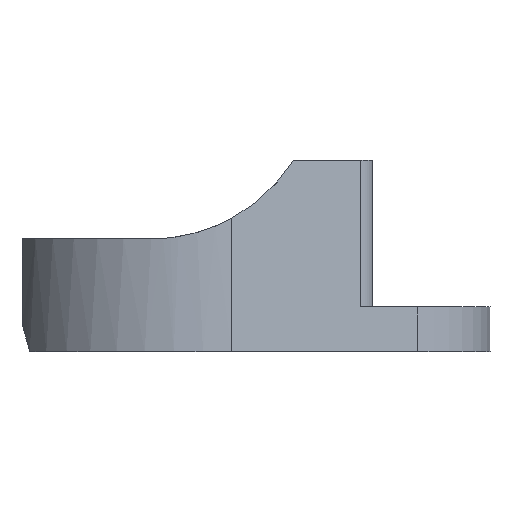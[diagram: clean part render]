
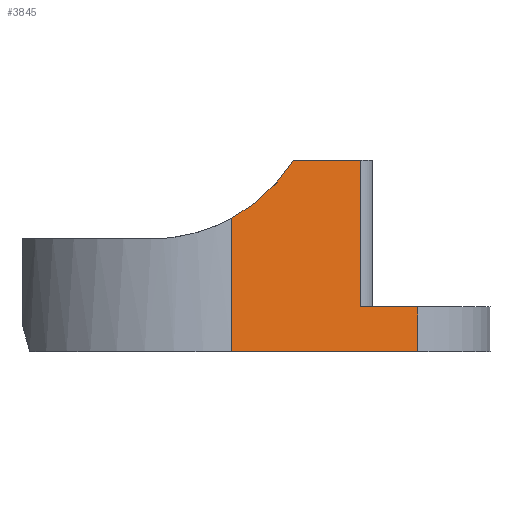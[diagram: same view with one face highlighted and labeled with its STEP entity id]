
A CAD part, left-side view. The second image highlights one B-rep face of the part: STEP entity #3845.
In plain terms, the highlighted planar face has unit normal (-0.95, -0.313, 0).
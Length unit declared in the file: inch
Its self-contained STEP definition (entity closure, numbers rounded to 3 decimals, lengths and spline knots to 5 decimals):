
#23=ELLIPSE('',#4035,0.78969,0.75);
#34=PLANE('',#4072);
#264=FACE_OUTER_BOUND('',#473,.T.);
#473=EDGE_LOOP('',(#3395,#3396,#3397,#3398,#3399,#3400,#3401));
#1074=LINE('',#12068,#1229);
#1077=LINE('',#16087,#1232);
#1079=LINE('',#16093,#1234);
#1080=LINE('',#16094,#1235);
#1081=LINE('',#16095,#1236);
#1082=LINE('',#16096,#1237);
#1229=VECTOR('',#4589,0.3937);
#1232=VECTOR('',#4628,0.3937);
#1234=VECTOR('',#4634,0.3937);
#1235=VECTOR('',#4635,0.3937);
#1236=VECTOR('',#4636,0.3937);
#1237=VECTOR('',#4637,0.3937);
#1628=VERTEX_POINT('',#11942);
#1629=VERTEX_POINT('',#11951);
#1638=VERTEX_POINT('',#12065);
#1639=VERTEX_POINT('',#12067);
#1644=VERTEX_POINT('',#16084);
#1645=VERTEX_POINT('',#16086);
#1647=VERTEX_POINT('',#16092);
#2174=EDGE_CURVE('',#1628,#1629,#23,.T.);
#2200=EDGE_CURVE('',#1638,#1639,#1074,.T.);
#2239=EDGE_CURVE('',#1644,#1645,#1077,.T.);
#2242=EDGE_CURVE('',#1645,#1647,#1079,.T.);
#2243=EDGE_CURVE('',#1629,#1644,#1080,.T.);
#2244=EDGE_CURVE('',#1639,#1628,#1081,.T.);
#2245=EDGE_CURVE('',#1638,#1647,#1082,.T.);
#3395=ORIENTED_EDGE('',*,*,#2242,.F.);
#3396=ORIENTED_EDGE('',*,*,#2239,.F.);
#3397=ORIENTED_EDGE('',*,*,#2243,.F.);
#3398=ORIENTED_EDGE('',*,*,#2174,.F.);
#3399=ORIENTED_EDGE('',*,*,#2244,.F.);
#3400=ORIENTED_EDGE('',*,*,#2200,.F.);
#3401=ORIENTED_EDGE('',*,*,#2245,.T.);
#3845=ADVANCED_FACE('',(#264),#34,.F.);
#4035=AXIS2_PLACEMENT_3D('',#11952,#4549,#4550);
#4072=AXIS2_PLACEMENT_3D('',#16091,#4632,#4633);
#4549=DIRECTION('center_axis',(-0.95,-0.313,0.));
#4550=DIRECTION('ref_axis',(0.313,-0.95,0.));
#4589=DIRECTION('',(-0.313,0.95,0.));
#4628=DIRECTION('',(0.,0.,-1.));
#4632=DIRECTION('center_axis',(0.95,0.313,0.));
#4633=DIRECTION('ref_axis',(-0.313,0.95,0.));
#4634=DIRECTION('',(0.313,-0.95,0.));
#4635=DIRECTION('',(0.313,-0.95,0.));
#4636=DIRECTION('',(0.,0.,1.));
#4637=DIRECTION('',(0.,0.,1.));
#11942=CARTESIAN_POINT('',(-0.7199,0.62771,-0.25889));
#11951=CARTESIAN_POINT('',(-0.62888,0.35157,0.));
#11952=CARTESIAN_POINT('Origin',(-0.838,0.986,0.4));
#12065=CARTESIAN_POINT('',(-0.44638,-0.20213,-0.853));
#12067=CARTESIAN_POINT('',(-0.7199,0.62771,-0.853));
#12068=CARTESIAN_POINT('',(-0.37651,-0.4141,-0.853));
#16084=CARTESIAN_POINT('',(-0.53044,0.0529,0.));
#16086=CARTESIAN_POINT('',(-0.53044,0.0529,-0.653));
#16087=CARTESIAN_POINT('',(-0.53044,0.0529,-0.4265));
#16091=CARTESIAN_POINT('Origin',(-0.44638,-0.20213,
-0.853));
#16092=CARTESIAN_POINT('',(-0.44638,-0.20213,-0.653));
#16093=CARTESIAN_POINT('',(-0.45455,-0.17733,-0.653));
#16094=CARTESIAN_POINT('',(-0.50682,-0.01877,0.));
#16095=CARTESIAN_POINT('',(-0.7199,0.62771,-0.853));
#16096=CARTESIAN_POINT('',(-0.44638,-0.20213,-0.853));
